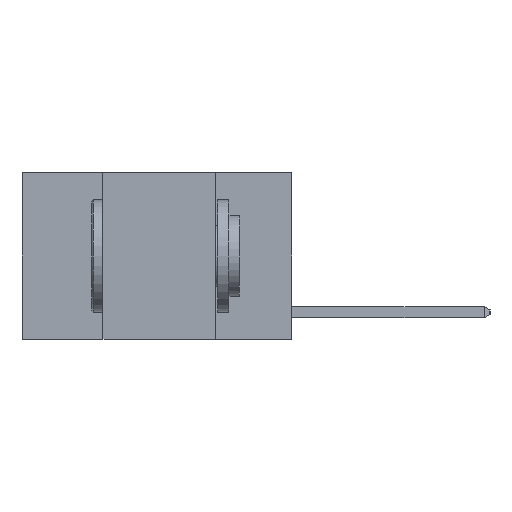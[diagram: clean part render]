
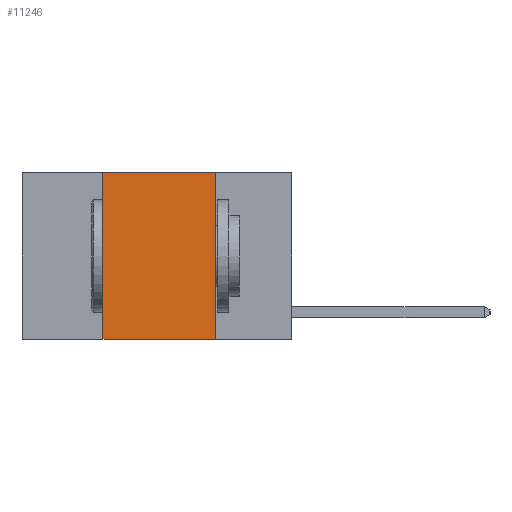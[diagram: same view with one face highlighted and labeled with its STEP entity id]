
A CAD part, left-side view. The second image highlights one B-rep face of the part: STEP entity #11246.
In plain terms, the highlighted planar face has unit normal (-1, 0, 0).
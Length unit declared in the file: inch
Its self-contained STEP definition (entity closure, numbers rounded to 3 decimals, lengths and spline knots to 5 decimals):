
#262 = CARTESIAN_POINT ( 'NONE',  ( 0., 0.42, -0.37 ) ) ;
#357 = ORIENTED_EDGE ( 'NONE', *, *, #5796, .F. ) ;
#599 = VECTOR ( 'NONE', #1884, 39.37008 ) ;
#790 = EDGE_CURVE ( 'NONE', #4423, #7916, #6546, .T. ) ;
#1161 = LINE ( 'NONE', #5921, #8428 ) ;
#1636 = VECTOR ( 'NONE', #2043, 39.37008 ) ;
#1884 = DIRECTION ( 'NONE',  ( 0., 0., 1. ) ) ;
#2043 = DIRECTION ( 'NONE',  ( 0., -1., 0. ) ) ;
#2465 = EDGE_CURVE ( 'NONE', #9000, #7916, #1161, .T. ) ;
#3317 = CARTESIAN_POINT ( 'NONE',  ( 0., 0.42, 0. ) ) ;
#3920 = VERTEX_POINT ( 'NONE', #3317 ) ;
#4075 = CARTESIAN_POINT ( 'NONE',  ( 0., 0.17, 0. ) ) ;
#4211 = PLANE ( 'NONE',  #9856 ) ;
#4423 = VERTEX_POINT ( 'NONE', #262 ) ;
#4646 = CARTESIAN_POINT ( 'NONE',  ( 0., 0.42, 0. ) ) ;
#5156 = DIRECTION ( 'NONE',  ( 1., 0., 0. ) ) ;
#5796 = EDGE_CURVE ( 'NONE', #4423, #3920, #9982, .T. ) ;
#5921 = CARTESIAN_POINT ( 'NONE',  ( 0., 0.17, 0. ) ) ;
#6060 = CARTESIAN_POINT ( 'NONE',  ( 0., 0.17, -0.37 ) ) ;
#6201 = ORIENTED_EDGE ( 'NONE', *, *, #790, .T. ) ;
#6546 = LINE ( 'NONE', #7464, #1636 ) ;
#6831 = DIRECTION ( 'NONE',  ( 0., 0., -1. ) ) ;
#7198 = LINE ( 'NONE', #9107, #9248 ) ;
#7464 = CARTESIAN_POINT ( 'NONE',  ( 0., 0.6, -0.37 ) ) ;
#7916 = VERTEX_POINT ( 'NONE', #6060 ) ;
#8042 = ORIENTED_EDGE ( 'NONE', *, *, #2465, .F. ) ;
#8317 = ORIENTED_EDGE ( 'NONE', *, *, #11595, .F. ) ;
#8428 = VECTOR ( 'NONE', #6831, 39.37008 ) ;
#9000 = VERTEX_POINT ( 'NONE', #4075 ) ;
#9107 = CARTESIAN_POINT ( 'NONE',  ( 0., 0.6, 0. ) ) ;
#9248 = VECTOR ( 'NONE', #9983, 39.37008 ) ;
#9856 = AXIS2_PLACEMENT_3D ( 'NONE', #10468, #5156, #11373 ) ;
#9982 = LINE ( 'NONE', #4646, #599 ) ;
#9983 = DIRECTION ( 'NONE',  ( 0., -1., 0. ) ) ;
#10215 = FACE_OUTER_BOUND ( 'NONE', #10779, .T. ) ;
#10468 = CARTESIAN_POINT ( 'NONE',  ( 0., 0.6, 0. ) ) ;
#10779 = EDGE_LOOP ( 'NONE', ( #8042, #8317, #357, #6201 ) ) ;
#11246 = ADVANCED_FACE ( 'NONE', ( #10215 ), #4211, .F. ) ;
#11373 = DIRECTION ( 'NONE',  ( 0., 0., -1. ) ) ;
#11595 = EDGE_CURVE ( 'NONE', #3920, #9000, #7198, .T. ) ;
